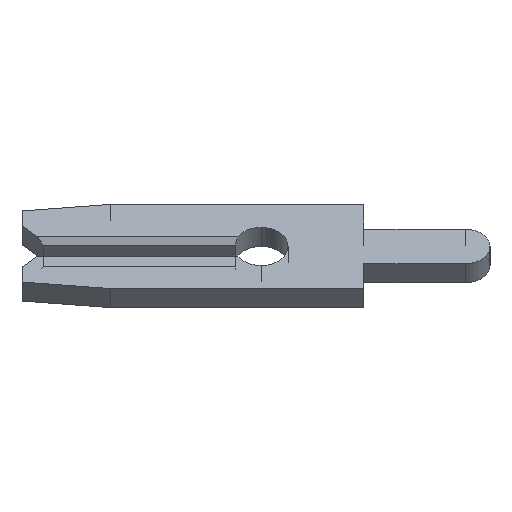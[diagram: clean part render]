
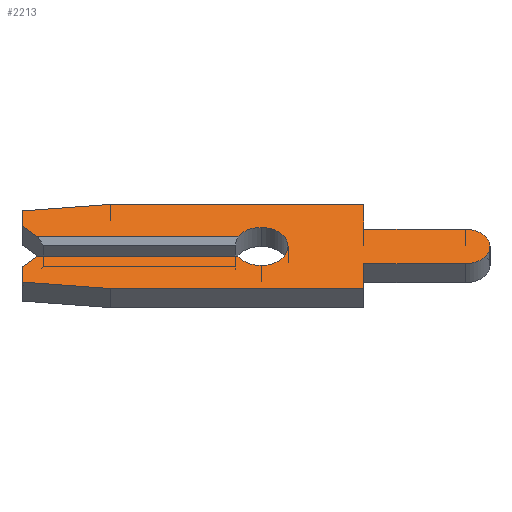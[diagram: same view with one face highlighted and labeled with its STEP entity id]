
A CAD part, left-side view. The second image highlights one B-rep face of the part: STEP entity #2213.
In plain terms, the highlighted face is planar.
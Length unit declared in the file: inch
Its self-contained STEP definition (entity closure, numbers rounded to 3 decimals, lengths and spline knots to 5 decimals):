
#2 = VERTEX_POINT ( 'NONE', #504 ) ;
#7 = CARTESIAN_POINT ( 'NONE',  ( -0.013, 0.216, 0.013 ) ) ;
#19 = CARTESIAN_POINT ( 'NONE',  ( -0.013, 0.231, -0.028 ) ) ;
#58 = CARTESIAN_POINT ( 'NONE',  ( -0.013, -0.099, -0.0575 ) ) ;
#83 = AXIS2_PLACEMENT_3D ( 'NONE', #1758, #1384, #2113 ) ;
#87 = DIRECTION ( 'NONE',  ( 0., 0., 1. ) ) ;
#104 = CARTESIAN_POINT ( 'NONE',  ( -0.013, -0.1975, 0. ) ) ;
#109 = EDGE_CURVE ( 'NONE', #1651, #2, #708, .T. ) ;
#145 = LINE ( 'NONE', #1083, #862 ) ;
#153 = ORIENTED_EDGE ( 'NONE', *, *, #2057, .F. ) ;
#162 = ORIENTED_EDGE ( 'NONE', *, *, #933, .F. ) ;
#176 = CARTESIAN_POINT ( 'NONE',  ( -0.013, 0.2105, 0.0075 ) ) ;
#183 = EDGE_CURVE ( 'NONE', #2, #1838, #841, .T. ) ;
#203 = AXIS2_PLACEMENT_3D ( 'NONE', #1422, #1942, #372 ) ;
#210 = ORIENTED_EDGE ( 'NONE', *, *, #1193, .F. ) ;
#232 = EDGE_CURVE ( 'NONE', #839, #2119, #1827, .T. ) ;
#265 = ORIENTED_EDGE ( 'NONE', *, *, #2101, .F. ) ;
#301 = EDGE_CURVE ( 'NONE', #1429, #1364, #1906, .T. ) ;
#325 = DIRECTION ( 'NONE',  ( 0., 1., 0. ) ) ;
#330 = CARTESIAN_POINT ( 'NONE',  ( -0.013, 0.231, 0.028 ) ) ;
#358 = DIRECTION ( 'NONE',  ( 0., -0.995, 0.105 ) ) ;
#363 = ORIENTED_EDGE ( 'NONE', *, *, #109, .F. ) ;
#369 = PLANE ( 'NONE',  #83 ) ;
#372 = DIRECTION ( 'NONE',  ( 0., 0., -1. ) ) ;
#373 = EDGE_CURVE ( 'NONE', #1364, #1455, #779, .T. ) ;
#400 = VECTOR ( 'NONE', #533, 39.37008 ) ;
#454 = CARTESIAN_POINT ( 'NONE',  ( -0.013, 0.231, 0.04857 ) ) ;
#460 = CARTESIAN_POINT ( 'NONE',  ( -0.013, 0.146, 0.0575 ) ) ;
#463 = ORIENTED_EDGE ( 'NONE', *, *, #616, .T. ) ;
#467 = CARTESIAN_POINT ( 'NONE',  ( -0.013, -0.099, 0.0575 ) ) ;
#471 = ORIENTED_EDGE ( 'NONE', *, *, #890, .F. ) ;
#491 = CARTESIAN_POINT ( 'NONE',  ( -0.013, 0.146, -0.0575 ) ) ;
#504 = CARTESIAN_POINT ( 'NONE',  ( -0.013, 0.02252, -0.013 ) ) ;
#511 = VECTOR ( 'NONE', #1547, 39.37008 ) ;
#515 = ORIENTED_EDGE ( 'NONE', *, *, #814, .F. ) ;
#533 = DIRECTION ( 'NONE',  ( 0., 0., 1. ) ) ;
#538 = VECTOR ( 'NONE', #1518, 39.37008 ) ;
#549 = VERTEX_POINT ( 'NONE', #1935 ) ;
#558 = EDGE_CURVE ( 'NONE', #2040, #669, #1067, .T. ) ;
#566 = VECTOR ( 'NONE', #1142, 39.37008 ) ;
#568 = ORIENTED_EDGE ( 'NONE', *, *, #183, .F. ) ;
#616 = EDGE_CURVE ( 'NONE', #2040, #1365, #145, .T. ) ;
#631 = VERTEX_POINT ( 'NONE', #888 ) ;
#632 = AXIS2_PLACEMENT_3D ( 'NONE', #104, #987, #87 ) ;
#639 = CARTESIAN_POINT ( 'NONE',  ( -0.013, 0.02252, 0.013 ) ) ;
#646 = DIRECTION ( 'NONE',  ( -1., 0., 0. ) ) ;
#668 = CARTESIAN_POINT ( 'NONE',  ( -0.013, -0.099, -0.0235 ) ) ;
#669 = VERTEX_POINT ( 'NONE', #1950 ) ;
#695 = CARTESIAN_POINT ( 'NONE',  ( -0.013, -0.099, -0.0235 ) ) ;
#708 = LINE ( 'NONE', #2209, #2171 ) ;
#720 = CARTESIAN_POINT ( 'NONE',  ( -0.013, -0.1975, -0.0235 ) ) ;
#743 = VERTEX_POINT ( 'NONE', #1780 ) ;
#779 = LINE ( 'NONE', #1573, #511 ) ;
#780 = DIRECTION ( 'NONE',  ( 0., 0.995, 0.105 ) ) ;
#793 = EDGE_LOOP ( 'NONE', ( #463, #515, #1486, #568, #363, #265, #153, #162, #1134, #471, #1559, #1340, #210, #1296, #1091, #1870, #1512, #1902 ) ) ;
#812 = DIRECTION ( 'NONE',  ( -1., 0., 0. ) ) ;
#814 = EDGE_CURVE ( 'NONE', #631, #1365, #2145, .T. ) ;
#827 = VERTEX_POINT ( 'NONE', #1788 ) ;
#837 = LINE ( 'NONE', #330, #889 ) ;
#839 = VERTEX_POINT ( 'NONE', #720 ) ;
#841 = CIRCLE ( 'NONE', #1288, 0.026 ) ;
#862 = VECTOR ( 'NONE', #1068, 39.37008 ) ;
#888 = CARTESIAN_POINT ( 'NONE',  ( -0.013, 0., 0.026 ) ) ;
#889 = VECTOR ( 'NONE', #1333, 39.37008 ) ;
#890 = EDGE_CURVE ( 'NONE', #2119, #743, #1177, .T. ) ;
#895 = VECTOR ( 'NONE', #358, 39.37008 ) ;
#919 = VECTOR ( 'NONE', #1394, 39.37008 ) ;
#933 = EDGE_CURVE ( 'NONE', #549, #1599, #2062, .T. ) ;
#948 = DIRECTION ( 'NONE',  ( 0., 0., -1. ) ) ;
#987 = DIRECTION ( 'NONE',  ( 1., 0., 0. ) ) ;
#1058 = CARTESIAN_POINT ( 'NONE',  ( -0.013, -0.099, 0.0235 ) ) ;
#1067 = LINE ( 'NONE', #176, #1310 ) ;
#1068 = DIRECTION ( 'NONE',  ( 0., -1., 0. ) ) ;
#1083 = CARTESIAN_POINT ( 'NONE',  ( -0.013, 0.231, 0.013 ) ) ;
#1091 = ORIENTED_EDGE ( 'NONE', *, *, #373, .F. ) ;
#1094 = FACE_OUTER_BOUND ( 'NONE', #793, .T. ) ;
#1111 = DIRECTION ( 'NONE',  ( 0., 0.707, 0.707 ) ) ;
#1119 = VECTOR ( 'NONE', #780, 39.37008 ) ;
#1134 = ORIENTED_EDGE ( 'NONE', *, *, #1687, .F. ) ;
#1142 = DIRECTION ( 'NONE',  ( 0., 0., -1. ) ) ;
#1151 = EDGE_CURVE ( 'NONE', #1838, #631, #2064, .T. ) ;
#1156 = CARTESIAN_POINT ( 'NONE',  ( -0.013, 0., 0. ) ) ;
#1169 = EDGE_CURVE ( 'NONE', #827, #839, #1366, .T. ) ;
#1177 = LINE ( 'NONE', #58, #1703 ) ;
#1193 = EDGE_CURVE ( 'NONE', #2165, #827, #2007, .T. ) ;
#1288 = AXIS2_PLACEMENT_3D ( 'NONE', #1540, #646, #1341 ) ;
#1296 = ORIENTED_EDGE ( 'NONE', *, *, #1388, .F. ) ;
#1310 = VECTOR ( 'NONE', #1111, 39.37008 ) ;
#1330 = CARTESIAN_POINT ( 'NONE',  ( -0.013, -0.099, 0.0575 ) ) ;
#1333 = DIRECTION ( 'NONE',  ( 0., 0., 1. ) ) ;
#1340 = ORIENTED_EDGE ( 'NONE', *, *, #1169, .F. ) ;
#1341 = DIRECTION ( 'NONE',  ( 0., 0., -1. ) ) ;
#1364 = VERTEX_POINT ( 'NONE', #460 ) ;
#1365 = VERTEX_POINT ( 'NONE', #639 ) ;
#1366 = CIRCLE ( 'NONE', #632, 0.0235 ) ;
#1384 = DIRECTION ( 'NONE',  ( 1., 0., 0. ) ) ;
#1388 = EDGE_CURVE ( 'NONE', #1455, #2165, #1674, .T. ) ;
#1394 = DIRECTION ( 'NONE',  ( 0., -0.707, 0.707 ) ) ;
#1411 = CARTESIAN_POINT ( 'NONE',  ( -0.013, 0.2105, -0.0075 ) ) ;
#1422 = CARTESIAN_POINT ( 'NONE',  ( -0.013, 0., 0. ) ) ;
#1429 = VERTEX_POINT ( 'NONE', #454 ) ;
#1455 = VERTEX_POINT ( 'NONE', #1330 ) ;
#1486 = ORIENTED_EDGE ( 'NONE', *, *, #1151, .F. ) ;
#1508 = LINE ( 'NONE', #491, #538 ) ;
#1512 = ORIENTED_EDGE ( 'NONE', *, *, #1787, .F. ) ;
#1518 = DIRECTION ( 'NONE',  ( 0., 1., 0. ) ) ;
#1522 = DIRECTION ( 'NONE',  ( 0., -1., 0. ) ) ;
#1527 = AXIS2_PLACEMENT_3D ( 'NONE', #1156, #812, #1656 ) ;
#1540 = CARTESIAN_POINT ( 'NONE',  ( -0.013, 0., 0. ) ) ;
#1542 = VECTOR ( 'NONE', #1851, 39.37008 ) ;
#1547 = DIRECTION ( 'NONE',  ( 0., -1., 0. ) ) ;
#1559 = ORIENTED_EDGE ( 'NONE', *, *, #232, .F. ) ;
#1573 = CARTESIAN_POINT ( 'NONE',  ( -0.013, 0.146, 0.0575 ) ) ;
#1599 = VERTEX_POINT ( 'NONE', #1868 ) ;
#1651 = VERTEX_POINT ( 'NONE', #2142 ) ;
#1656 = DIRECTION ( 'NONE',  ( 0., 0., -1. ) ) ;
#1674 = LINE ( 'NONE', #467, #566 ) ;
#1687 = EDGE_CURVE ( 'NONE', #743, #549, #1508, .T. ) ;
#1688 = CARTESIAN_POINT ( 'NONE',  ( -0.013, -0.099, 0.0235 ) ) ;
#1703 = VECTOR ( 'NONE', #948, 39.37008 ) ;
#1730 = CARTESIAN_POINT ( 'NONE',  ( -0.013, 0.231, 0.04857 ) ) ;
#1749 = CARTESIAN_POINT ( 'NONE',  ( -0.013, 0.231, -0.028 ) ) ;
#1758 = CARTESIAN_POINT ( 'NONE',  ( -0.013, 0., 0. ) ) ;
#1780 = CARTESIAN_POINT ( 'NONE',  ( -0.013, -0.099, -0.0575 ) ) ;
#1787 = EDGE_CURVE ( 'NONE', #669, #1429, #837, .T. ) ;
#1788 = CARTESIAN_POINT ( 'NONE',  ( -0.013, -0.1975, 0.0235 ) ) ;
#1800 = CARTESIAN_POINT ( 'NONE',  ( -0.013, 0.231, -0.04857 ) ) ;
#1827 = LINE ( 'NONE', #668, #2013 ) ;
#1838 = VERTEX_POINT ( 'NONE', #2218 ) ;
#1851 = DIRECTION ( 'NONE',  ( 0., -1., 0. ) ) ;
#1868 = CARTESIAN_POINT ( 'NONE',  ( -0.013, 0.231, -0.04857 ) ) ;
#1870 = ORIENTED_EDGE ( 'NONE', *, *, #301, .F. ) ;
#1898 = LINE ( 'NONE', #1749, #400 ) ;
#1902 = ORIENTED_EDGE ( 'NONE', *, *, #558, .F. ) ;
#1906 = LINE ( 'NONE', #1730, #895 ) ;
#1935 = CARTESIAN_POINT ( 'NONE',  ( -0.013, 0.146, -0.0575 ) ) ;
#1942 = DIRECTION ( 'NONE',  ( -1., 0., 0. ) ) ;
#1950 = CARTESIAN_POINT ( 'NONE',  ( -0.013, 0.231, 0.028 ) ) ;
#2007 = LINE ( 'NONE', #1688, #1542 ) ;
#2013 = VECTOR ( 'NONE', #325, 39.37008 ) ;
#2040 = VERTEX_POINT ( 'NONE', #7 ) ;
#2057 = EDGE_CURVE ( 'NONE', #1599, #2132, #1898, .T. ) ;
#2062 = LINE ( 'NONE', #1800, #1119 ) ;
#2064 = CIRCLE ( 'NONE', #1527, 0.026 ) ;
#2091 = LINE ( 'NONE', #1411, #919 ) ;
#2101 = EDGE_CURVE ( 'NONE', #2132, #1651, #2091, .T. ) ;
#2113 = DIRECTION ( 'NONE',  ( 0., 0., -1. ) ) ;
#2119 = VERTEX_POINT ( 'NONE', #695 ) ;
#2132 = VERTEX_POINT ( 'NONE', #19 ) ;
#2142 = CARTESIAN_POINT ( 'NONE',  ( -0.013, 0.216, -0.013 ) ) ;
#2145 = CIRCLE ( 'NONE', #203, 0.026 ) ;
#2165 = VERTEX_POINT ( 'NONE', #1058 ) ;
#2171 = VECTOR ( 'NONE', #1522, 39.37008 ) ;
#2209 = CARTESIAN_POINT ( 'NONE',  ( -0.013, 0., -0.013 ) ) ;
#2213 = ADVANCED_FACE ( 'NONE', ( #1094 ), #369, .F. ) ;
#2218 = CARTESIAN_POINT ( 'NONE',  ( -0.013, 0., -0.026 ) ) ;
